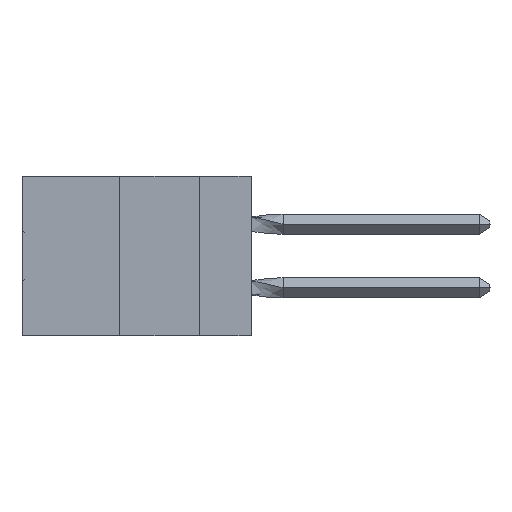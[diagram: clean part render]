
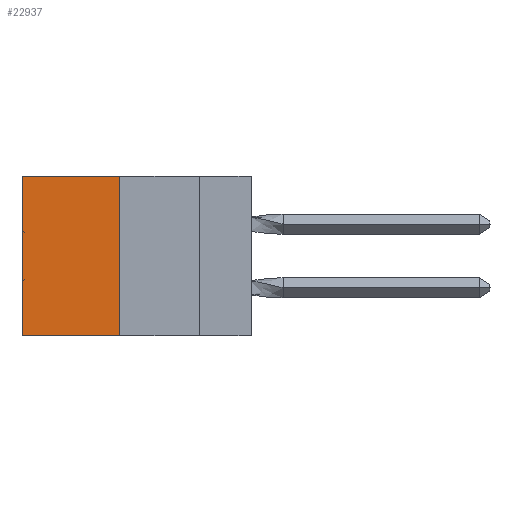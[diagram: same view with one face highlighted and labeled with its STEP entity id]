
A CAD part, left-side view. The second image highlights one B-rep face of the part: STEP entity #22937.
In plain terms, the highlighted planar face has unit normal (-1, 0, 0).
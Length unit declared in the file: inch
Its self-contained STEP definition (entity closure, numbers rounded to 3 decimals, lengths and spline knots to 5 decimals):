
#1008 = CARTESIAN_POINT ( 'NONE',  ( 0.305, 0.413, -0.5 ) ) ;
#1748 = FACE_OUTER_BOUND ( 'NONE', #28044, .T. ) ;
#4925 = VERTEX_POINT ( 'NONE', #15020 ) ;
#8612 = VERTEX_POINT ( 'NONE', #30343 ) ;
#9350 = AXIS2_PLACEMENT_3D ( 'NONE', #37191, #29647, #14575 ) ;
#10636 = ORIENTED_EDGE ( 'NONE', *, *, #34396, .T. ) ;
#12923 = CARTESIAN_POINT ( 'NONE',  ( 0.305, 0.413, 0. ) ) ;
#14140 = LINE ( 'NONE', #19911, #21869 ) ;
#14575 = DIRECTION ( 'NONE',  ( 0., 0., -1. ) ) ;
#14751 = VERTEX_POINT ( 'NONE', #12923 ) ;
#15020 = CARTESIAN_POINT ( 'NONE',  ( 0.305, 0.413, -0.5 ) ) ;
#15964 = CARTESIAN_POINT ( 'NONE',  ( 0.305, 0.72, 0. ) ) ;
#16082 = VECTOR ( 'NONE', #22726, 39.37008 ) ;
#16323 = EDGE_CURVE ( 'NONE', #14751, #4925, #14140, .T. ) ;
#18230 = PLANE ( 'NONE',  #9350 ) ;
#18532 = ORIENTED_EDGE ( 'NONE', *, *, #16323, .F. ) ;
#19911 = CARTESIAN_POINT ( 'NONE',  ( 0.305, 0.413, -0.5 ) ) ;
#21869 = VECTOR ( 'NONE', #31192, 39.37008 ) ;
#22726 = DIRECTION ( 'NONE',  ( 0., 1., 0. ) ) ;
#22937 = ADVANCED_FACE ( 'NONE', ( #1748 ), #18230, .F. ) ;
#26130 = LINE ( 'NONE', #26518, #16082 ) ;
#26518 = CARTESIAN_POINT ( 'NONE',  ( 0.305, 0.413, 0. ) ) ;
#27767 = DIRECTION ( 'NONE',  ( 0., 1., 0. ) ) ;
#28044 = EDGE_LOOP ( 'NONE', ( #10636, #39911, #18532, #35303 ) ) ;
#29647 = DIRECTION ( 'NONE',  ( 1., 0., 0. ) ) ;
#30343 = CARTESIAN_POINT ( 'NONE',  ( 0.305, 0.72, -0.5 ) ) ;
#31192 = DIRECTION ( 'NONE',  ( 0., 0., -1. ) ) ;
#31322 = LINE ( 'NONE', #1008, #32485 ) ;
#31543 = EDGE_CURVE ( 'NONE', #14751, #41901, #26130, .T. ) ;
#32485 = VECTOR ( 'NONE', #27767, 39.37008 ) ;
#33993 = DIRECTION ( 'NONE',  ( 0., 0., -1. ) ) ;
#34186 = LINE ( 'NONE', #37501, #44906 ) ;
#34396 = EDGE_CURVE ( 'NONE', #41901, #8612, #34186, .T. ) ;
#35303 = ORIENTED_EDGE ( 'NONE', *, *, #31543, .T. ) ;
#37191 = CARTESIAN_POINT ( 'NONE',  ( 0.305, 0.413, -0.5 ) ) ;
#37501 = CARTESIAN_POINT ( 'NONE',  ( 0.305, 0.72, -0.5 ) ) ;
#39684 = EDGE_CURVE ( 'NONE', #4925, #8612, #31322, .T. ) ;
#39911 = ORIENTED_EDGE ( 'NONE', *, *, #39684, .F. ) ;
#41901 = VERTEX_POINT ( 'NONE', #15964 ) ;
#44906 = VECTOR ( 'NONE', #33993, 39.37008 ) ;
